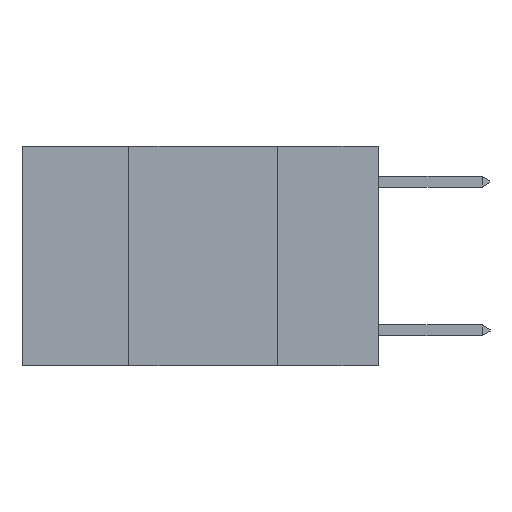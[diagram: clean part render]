
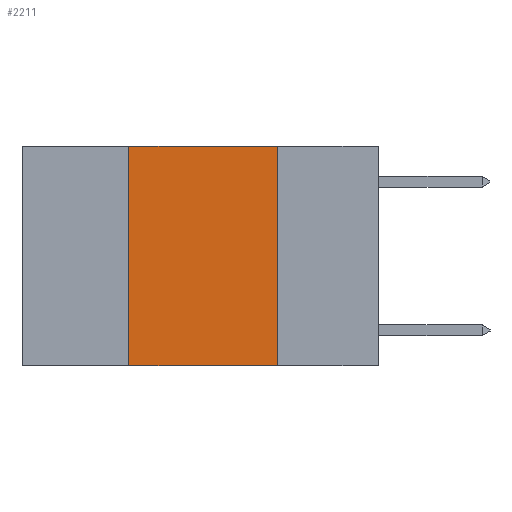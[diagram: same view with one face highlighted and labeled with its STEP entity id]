
A CAD part, left-side view. The second image highlights one B-rep face of the part: STEP entity #2211.
In plain terms, the highlighted planar face has unit normal (-1, 0, 0).
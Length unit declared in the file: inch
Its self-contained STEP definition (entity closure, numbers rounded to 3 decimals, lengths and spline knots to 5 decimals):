
#205 = EDGE_CURVE ( 'NONE', #6400, #8630, #6405, .T. ) ;
#254 = VECTOR ( 'NONE', #7855, 39.37008 ) ;
#473 = DIRECTION ( 'NONE',  ( 0., 0., -1. ) ) ;
#719 = DIRECTION ( 'NONE',  ( 0., 0., -1. ) ) ;
#960 = AXIS2_PLACEMENT_3D ( 'NONE', #3534, #5076, #473 ) ;
#1451 = VECTOR ( 'NONE', #719, 39.37008 ) ;
#1561 = DIRECTION ( 'NONE',  ( 0., -1., 0. ) ) ;
#2112 = FACE_OUTER_BOUND ( 'NONE', #4733, .T. ) ;
#2169 = ORIENTED_EDGE ( 'NONE', *, *, #205, .F. ) ;
#2211 = ADVANCED_FACE ( 'NONE', ( #2112 ), #9784, .F. ) ;
#2230 = CARTESIAN_POINT ( 'NONE',  ( 0., 0.42, 0. ) ) ;
#2346 = VERTEX_POINT ( 'NONE', #5212 ) ;
#2381 = CARTESIAN_POINT ( 'NONE',  ( 0., 0.42, 0. ) ) ;
#2536 = CARTESIAN_POINT ( 'NONE',  ( 0., 0.42, -0.37 ) ) ;
#2800 = ORIENTED_EDGE ( 'NONE', *, *, #3754, .T. ) ;
#3534 = CARTESIAN_POINT ( 'NONE',  ( 0., 0.6, 0. ) ) ;
#3588 = CARTESIAN_POINT ( 'NONE',  ( 0., 0.6, 0. ) ) ;
#3754 = EDGE_CURVE ( 'NONE', #6400, #2346, #9434, .T. ) ;
#3864 = ORIENTED_EDGE ( 'NONE', *, *, #7962, .F. ) ;
#4496 = CARTESIAN_POINT ( 'NONE',  ( 0., 0.17, 0. ) ) ;
#4733 = EDGE_LOOP ( 'NONE', ( #3864, #8648, #2169, #2800 ) ) ;
#5076 = DIRECTION ( 'NONE',  ( 1., 0., 0. ) ) ;
#5212 = CARTESIAN_POINT ( 'NONE',  ( 0., 0.17, -0.37 ) ) ;
#5513 = VECTOR ( 'NONE', #1561, 39.37008 ) ;
#6185 = CARTESIAN_POINT ( 'NONE',  ( 0., 0.6, -0.37 ) ) ;
#6400 = VERTEX_POINT ( 'NONE', #2536 ) ;
#6405 = LINE ( 'NONE', #2381, #254 ) ;
#7257 = EDGE_CURVE ( 'NONE', #8630, #9218, #9621, .T. ) ;
#7513 = VECTOR ( 'NONE', #8234, 39.37008 ) ;
#7855 = DIRECTION ( 'NONE',  ( 0., 0., 1. ) ) ;
#7962 = EDGE_CURVE ( 'NONE', #9218, #2346, #8121, .T. ) ;
#8121 = LINE ( 'NONE', #4496, #1451 ) ;
#8234 = DIRECTION ( 'NONE',  ( 0., -1., 0. ) ) ;
#8630 = VERTEX_POINT ( 'NONE', #2230 ) ;
#8648 = ORIENTED_EDGE ( 'NONE', *, *, #7257, .F. ) ;
#9199 = CARTESIAN_POINT ( 'NONE',  ( 0., 0.17, 0. ) ) ;
#9218 = VERTEX_POINT ( 'NONE', #9199 ) ;
#9434 = LINE ( 'NONE', #6185, #5513 ) ;
#9621 = LINE ( 'NONE', #3588, #7513 ) ;
#9784 = PLANE ( 'NONE',  #960 ) ;
